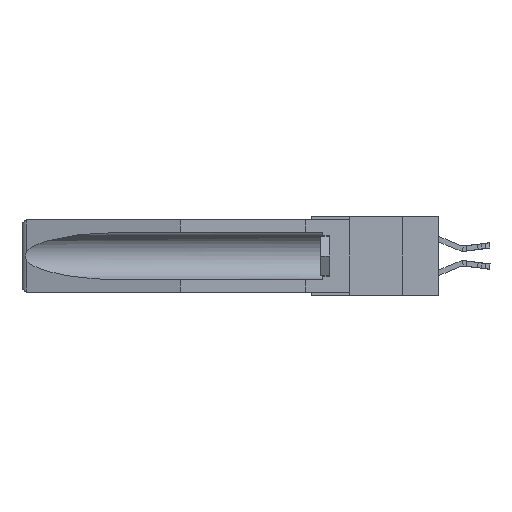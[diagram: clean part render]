
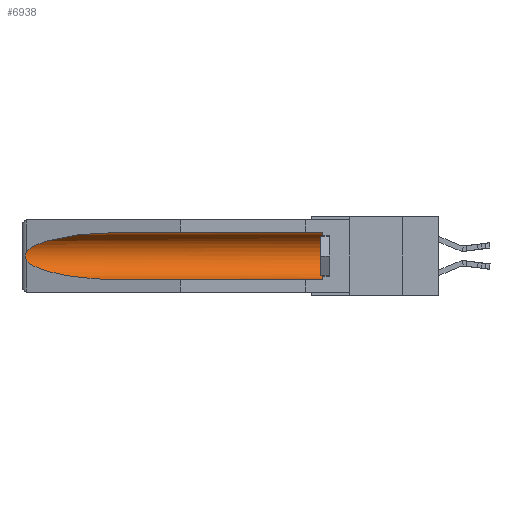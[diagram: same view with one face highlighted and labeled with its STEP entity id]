
A CAD part, left-side view. The second image highlights one B-rep face of the part: STEP entity #6938.
In plain terms, the highlighted cylindrical face has radius 2.857 mm (diameter 5.715 mm), a partial arc.
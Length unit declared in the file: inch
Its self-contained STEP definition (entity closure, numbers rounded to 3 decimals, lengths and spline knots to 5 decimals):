
#1102 = VERTEX_POINT ( 'NONE', #13359 ) ;
#1110 = ORIENTED_EDGE ( 'NONE', *, *, #13870, .F. ) ;
#2113 = CARTESIAN_POINT ( 'NONE',  ( 0.155, 0.126, -0.284 ) ) ;
#2162 = CARTESIAN_POINT ( 'NONE',  ( 0.26654, 1.53092, -0.15636 ) ) ;
#2200 = EDGE_CURVE ( 'NONE', #14513, #18470, #23467, .T. ) ;
#2262 = CARTESIAN_POINT ( 'NONE',  ( 0.21114, 1.30732, -0.284 ) ) ;
#2272 = CARTESIAN_POINT ( 'NONE',  ( 0.26537, 1.52718, -0.14972 ) ) ;
#2674 = CIRCLE ( 'NONE', #31228, 0.1125 ) ;
#3156 = DIRECTION ( 'NONE',  ( 0., 1., 0. ) ) ;
#3594 = CARTESIAN_POINT ( 'NONE',  ( 0.155, 1.07973, -0.284 ) ) ;
#4722 = CARTESIAN_POINT ( 'NONE',  ( 0.2673, 1.5327, -0.16383 ) ) ;
#4836 = CARTESIAN_POINT ( 'NONE',  ( 0.26597, 1.5296, -0.19026 ) ) ;
#5649 = AXIS2_PLACEMENT_3D ( 'NONE', #7736, #12918, #12483 ) ;
#6701 = CARTESIAN_POINT ( 'NONE',  ( 0.155, 1.07973, -0.059 ) ) ;
#6729 = CARTESIAN_POINT ( 'NONE',  ( 0.26537, 1.52718, -0.14972 ) ) ;
#6938 = ADVANCED_FACE ( 'NONE', ( #27911 ), #18006, .F. ) ;
#7736 = CARTESIAN_POINT ( 'NONE',  ( 0.155, -0.30754, -0.1715 ) ) ;
#8391 = CARTESIAN_POINT ( 'NONE',  ( 0.155, -0.30754, -0.059 ) ) ;
#9037 = CARTESIAN_POINT ( 'NONE',  ( 0.26537, 1.52718, -0.19328 ) ) ;
#9761 = LINE ( 'NONE', #30138, #27631 ) ;
#10780 = VERTEX_POINT ( 'NONE', #2113 ) ;
#11224 = CARTESIAN_POINT ( 'NONE',  ( 0.155, 0.126, -0.1715 ) ) ;
#12327 = DIRECTION ( 'NONE',  ( 0., 1., 0. ) ) ;
#12483 = DIRECTION ( 'NONE',  ( 0., 0., 1. ) ) ;
#12918 = DIRECTION ( 'NONE',  ( 0., 1., 0. ) ) ;
#13000 = EDGE_CURVE ( 'NONE', #10780, #1102, #2674, .T. ) ;
#13234 = ORIENTED_EDGE ( 'NONE', *, *, #22824, .T. ) ;
#13359 = CARTESIAN_POINT ( 'NONE',  ( 0.155, 0.126, -0.059 ) ) ;
#13844 = EDGE_CURVE ( 'NONE', #20365, #14513, #14075, .T. ) ;
#13870 = EDGE_CURVE ( 'NONE', #10780, #18654, #9761, .T. ) ;
#14075 =( BOUNDED_CURVE ( )  B_SPLINE_CURVE ( 3, ( #6701, #29484, #14321, #16995 ),
 .UNSPECIFIED., .F., .F. ) 
 B_SPLINE_CURVE_WITH_KNOTS ( ( 4, 4 ),
 ( 4.71239, 6.08839 ),
 .UNSPECIFIED. ) 
 CURVE ( )  GEOMETRIC_REPRESENTATION_ITEM ( )  RATIONAL_B_SPLINE_CURVE ( ( 1., 0.848, 0.848, 1. ) ) 
 REPRESENTATION_ITEM ( '' )  );
#14321 = CARTESIAN_POINT ( 'NONE',  ( 0.25451, 1.48313, -0.09465 ) ) ;
#14513 = VERTEX_POINT ( 'NONE', #6729 ) ;
#16292 = EDGE_CURVE ( 'NONE', #1102, #20365, #32034, .T. ) ;
#16995 = CARTESIAN_POINT ( 'NONE',  ( 0.26537, 1.52718, -0.14972 ) ) ;
#17245 = CARTESIAN_POINT ( 'NONE',  ( 0.155, 1.07973, -0.059 ) ) ;
#18006 = CYLINDRICAL_SURFACE ( 'NONE', #5649, 0.1125 ) ;
#18470 = VERTEX_POINT ( 'NONE', #29252 ) ;
#18654 = VERTEX_POINT ( 'NONE', #3594 ) ;
#19254 = ORIENTED_EDGE ( 'NONE', *, *, #13844, .T. ) ;
#19322 = ORIENTED_EDGE ( 'NONE', *, *, #13000, .T. ) ;
#19417 = ORIENTED_EDGE ( 'NONE', *, *, #16292, .T. ) ;
#19472 = CARTESIAN_POINT ( 'NONE',  ( 0.155, 1.07973, -0.284 ) ) ;
#19557 =( BOUNDED_CURVE ( )  B_SPLINE_CURVE ( 3, ( #9037, #29504, #2262, #19472 ),
 .UNSPECIFIED., .F., .F. ) 
 B_SPLINE_CURVE_WITH_KNOTS ( ( 4, 4 ),
 ( 0.1948, 1.5708 ),
 .UNSPECIFIED. ) 
 CURVE ( )  GEOMETRIC_REPRESENTATION_ITEM ( )  RATIONAL_B_SPLINE_CURVE ( ( 1., 0.848, 0.848, 1. ) ) 
 REPRESENTATION_ITEM ( '' )  );
#20365 = VERTEX_POINT ( 'NONE', #17245 ) ;
#22484 = CARTESIAN_POINT ( 'NONE',  ( 0.2675, 1.53308, -0.17534 ) ) ;
#22595 = CARTESIAN_POINT ( 'NONE',  ( 0.26537, 1.52718, -0.19328 ) ) ;
#22824 = EDGE_CURVE ( 'NONE', #18470, #18654, #19557, .T. ) ;
#23467 = B_SPLINE_CURVE_WITH_KNOTS ( 'NONE', 3,
 ( #2272, #32555, #2162, #4722, #32806, #22484, #30295, #25034, #4836, #22595 ),
 .UNSPECIFIED., .F., .F.,
 ( 4, 2, 2, 2, 4 ),
 ( 0., 0.00029, 0.00058, 0.00087, 0.00117 ),
 .UNSPECIFIED. ) ;
#25034 = CARTESIAN_POINT ( 'NONE',  ( 0.26655, 1.53094, -0.18657 ) ) ;
#25333 = VECTOR ( 'NONE', #3156, 39.37008 ) ;
#25979 = EDGE_LOOP ( 'NONE', ( #19254, #28462, #13234, #1110, #19322, #19417 ) ) ;
#26329 = DIRECTION ( 'NONE',  ( 0., 0., 1. ) ) ;
#26438 = DIRECTION ( 'NONE',  ( 0., -1., 0. ) ) ;
#27631 = VECTOR ( 'NONE', #12327, 39.37008 ) ;
#27911 = FACE_OUTER_BOUND ( 'NONE', #25979, .T. ) ;
#28462 = ORIENTED_EDGE ( 'NONE', *, *, #2200, .T. ) ;
#29252 = CARTESIAN_POINT ( 'NONE',  ( 0.26537, 1.52718, -0.19328 ) ) ;
#29484 = CARTESIAN_POINT ( 'NONE',  ( 0.21114, 1.30732, -0.059 ) ) ;
#29504 = CARTESIAN_POINT ( 'NONE',  ( 0.25451, 1.48313, -0.24835 ) ) ;
#30138 = CARTESIAN_POINT ( 'NONE',  ( 0.155, -0.30754, -0.284 ) ) ;
#30295 = CARTESIAN_POINT ( 'NONE',  ( 0.2673, 1.53269, -0.17917 ) ) ;
#31228 = AXIS2_PLACEMENT_3D ( 'NONE', #11224, #26438, #26329 ) ;
#32034 = LINE ( 'NONE', #8391, #25333 ) ;
#32555 = CARTESIAN_POINT ( 'NONE',  ( 0.26597, 1.52961, -0.15275 ) ) ;
#32806 = CARTESIAN_POINT ( 'NONE',  ( 0.2675, 1.53308, -0.16763 ) ) ;
